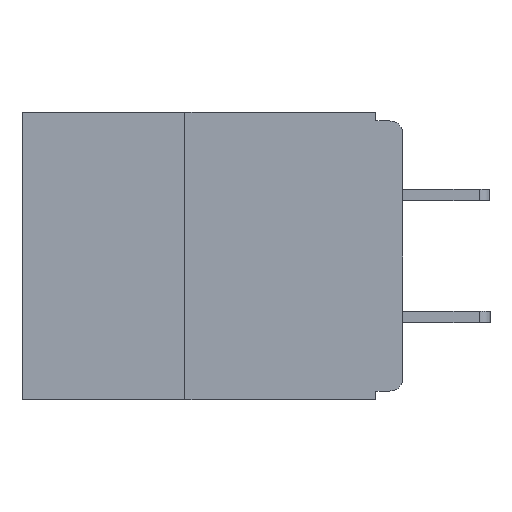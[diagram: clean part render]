
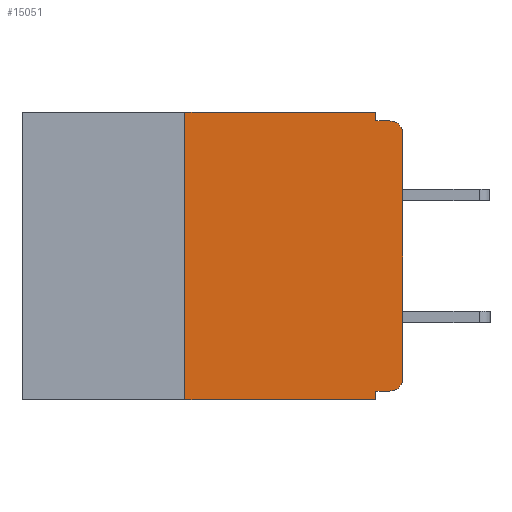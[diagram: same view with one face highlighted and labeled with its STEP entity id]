
A CAD part, left-side view. The second image highlights one B-rep face of the part: STEP entity #15051.
In plain terms, the highlighted planar face has unit normal (-1, 0, 0).
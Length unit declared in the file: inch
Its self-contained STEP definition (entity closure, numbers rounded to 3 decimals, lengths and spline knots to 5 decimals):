
#332 = CARTESIAN_POINT ( 'NONE',  ( 0., 0.031, -0.33 ) ) ;
#505 = CARTESIAN_POINT ( 'NONE',  ( 0., 0.015, -0.01 ) ) ;
#1168 = CARTESIAN_POINT ( 'NONE',  ( 0., 0.031, 0. ) ) ;
#1361 = ORIENTED_EDGE ( 'NONE', *, *, #12454, .T. ) ;
#1710 = VECTOR ( 'NONE', #12046, 39.37008 ) ;
#1731 = DIRECTION ( 'NONE',  ( -1., 0., 0. ) ) ;
#2186 = DIRECTION ( 'NONE',  ( 0., -1., 0. ) ) ;
#2817 = VERTEX_POINT ( 'NONE', #505 ) ;
#2874 = EDGE_CURVE ( 'NONE', #10611, #2817, #9341, .T. ) ;
#2976 = VERTEX_POINT ( 'NONE', #8326 ) ;
#3410 = LINE ( 'NONE', #15241, #10658 ) ;
#3461 = EDGE_CURVE ( 'NONE', #7447, #2817, #19648, .T. ) ;
#3481 = LINE ( 'NONE', #17397, #15344 ) ;
#3665 = CARTESIAN_POINT ( 'NONE',  ( 0., 0.25, 0. ) ) ;
#4322 = VERTEX_POINT ( 'NONE', #332 ) ;
#5037 = ORIENTED_EDGE ( 'NONE', *, *, #19252, .F. ) ;
#5082 = VECTOR ( 'NONE', #9387, 39.37008 ) ;
#5200 = LINE ( 'NONE', #10723, #17069 ) ;
#5267 = CARTESIAN_POINT ( 'NONE',  ( 0., 0.031, -0.33 ) ) ;
#5450 = CARTESIAN_POINT ( 'NONE',  ( 0., 0., -0.01 ) ) ;
#5561 = LINE ( 'NONE', #17117, #5082 ) ;
#5751 = EDGE_CURVE ( 'NONE', #2976, #15133, #3481, .T. ) ;
#5783 = VERTEX_POINT ( 'NONE', #3665 ) ;
#6056 = EDGE_CURVE ( 'NONE', #7244, #7447, #14625, .T. ) ;
#6333 = ORIENTED_EDGE ( 'NONE', *, *, #8469, .T. ) ;
#6437 = ORIENTED_EDGE ( 'NONE', *, *, #15261, .F. ) ;
#6460 = CARTESIAN_POINT ( 'NONE',  ( 0., 0., 0. ) ) ;
#6567 = CARTESIAN_POINT ( 'NONE',  ( 0., 0., -0.305 ) ) ;
#6750 = LINE ( 'NONE', #6460, #14561 ) ;
#6939 = ORIENTED_EDGE ( 'NONE', *, *, #3461, .F. ) ;
#7207 = CARTESIAN_POINT ( 'NONE',  ( 0., 0.031, 0. ) ) ;
#7244 = VERTEX_POINT ( 'NONE', #7207 ) ;
#7447 = VERTEX_POINT ( 'NONE', #18768 ) ;
#7630 = EDGE_CURVE ( 'NONE', #15133, #4322, #10176, .T. ) ;
#8180 = VERTEX_POINT ( 'NONE', #6567 ) ;
#8290 = AXIS2_PLACEMENT_3D ( 'NONE', #13359, #8723, #19452 ) ;
#8326 = CARTESIAN_POINT ( 'NONE',  ( 0., 0.015, -0.32 ) ) ;
#8469 = EDGE_CURVE ( 'NONE', #2976, #8180, #19533, .T. ) ;
#8721 = AXIS2_PLACEMENT_3D ( 'NONE', #19650, #13366, #12940 ) ;
#8723 = DIRECTION ( 'NONE',  ( 1., 0., 0. ) ) ;
#9241 = DIRECTION ( 'NONE',  ( 0., -1., 0. ) ) ;
#9341 = CIRCLE ( 'NONE', #8721, 0.015 ) ;
#9387 = DIRECTION ( 'NONE',  ( 0., -1., 0. ) ) ;
#10122 = ORIENTED_EDGE ( 'NONE', *, *, #6056, .F. ) ;
#10176 = LINE ( 'NONE', #5267, #17919 ) ;
#10611 = VERTEX_POINT ( 'NONE', #11671 ) ;
#10658 = VECTOR ( 'NONE', #13711, 39.37008 ) ;
#10723 = CARTESIAN_POINT ( 'NONE',  ( 0., 0.437, 0. ) ) ;
#11034 = CARTESIAN_POINT ( 'NONE',  ( 0., 0.015, -0.305 ) ) ;
#11171 = DIRECTION ( 'NONE',  ( 0., 0., 1. ) ) ;
#11434 = DIRECTION ( 'NONE',  ( 0., 0., -1. ) ) ;
#11671 = CARTESIAN_POINT ( 'NONE',  ( 0., 0., -0.025 ) ) ;
#12046 = DIRECTION ( 'NONE',  ( 0., 0., -1. ) ) ;
#12454 = EDGE_CURVE ( 'NONE', #15502, #4322, #5561, .T. ) ;
#12639 = DIRECTION ( 'NONE',  ( 0., 0., -1. ) ) ;
#12746 = DIRECTION ( 'NONE',  ( 0., 1., 0. ) ) ;
#12927 = CARTESIAN_POINT ( 'NONE',  ( 0., 0.25, -0.33 ) ) ;
#12940 = DIRECTION ( 'NONE',  ( 0., 0., -1. ) ) ;
#13359 = CARTESIAN_POINT ( 'NONE',  ( 0., 0.437, 0. ) ) ;
#13366 = DIRECTION ( 'NONE',  ( -1., 0., 0. ) ) ;
#13711 = DIRECTION ( 'NONE',  ( 0., 0., 1. ) ) ;
#14015 = ORIENTED_EDGE ( 'NONE', *, *, #7630, .F. ) ;
#14517 = EDGE_LOOP ( 'NONE', ( #19270, #16187, #6939, #10122, #6437, #5037, #1361, #14015, #19026, #6333 ) ) ;
#14561 = VECTOR ( 'NONE', #11171, 39.37008 ) ;
#14625 = LINE ( 'NONE', #1168, #1710 ) ;
#15051 = ADVANCED_FACE ( 'NONE', ( #16851 ), #16428, .F. ) ;
#15133 = VERTEX_POINT ( 'NONE', #16631 ) ;
#15153 = VECTOR ( 'NONE', #2186, 39.37008 ) ;
#15241 = CARTESIAN_POINT ( 'NONE',  ( 0., 0.25, -0.33 ) ) ;
#15261 = EDGE_CURVE ( 'NONE', #5783, #7244, #5200, .T. ) ;
#15344 = VECTOR ( 'NONE', #12746, 39.37008 ) ;
#15502 = VERTEX_POINT ( 'NONE', #12927 ) ;
#16187 = ORIENTED_EDGE ( 'NONE', *, *, #2874, .T. ) ;
#16428 = PLANE ( 'NONE',  #8290 ) ;
#16631 = CARTESIAN_POINT ( 'NONE',  ( 0., 0.031, -0.32 ) ) ;
#16851 = FACE_OUTER_BOUND ( 'NONE', #14517, .T. ) ;
#17069 = VECTOR ( 'NONE', #9241, 39.37008 ) ;
#17117 = CARTESIAN_POINT ( 'NONE',  ( 0., 0.437, -0.33 ) ) ;
#17397 = CARTESIAN_POINT ( 'NONE',  ( 0., 0., -0.32 ) ) ;
#17919 = VECTOR ( 'NONE', #11434, 39.37008 ) ;
#17974 = AXIS2_PLACEMENT_3D ( 'NONE', #11034, #1731, #12639 ) ;
#18768 = CARTESIAN_POINT ( 'NONE',  ( 0., 0.031, -0.01 ) ) ;
#18859 = EDGE_CURVE ( 'NONE', #8180, #10611, #6750, .T. ) ;
#19026 = ORIENTED_EDGE ( 'NONE', *, *, #5751, .F. ) ;
#19252 = EDGE_CURVE ( 'NONE', #15502, #5783, #3410, .T. ) ;
#19270 = ORIENTED_EDGE ( 'NONE', *, *, #18859, .T. ) ;
#19452 = DIRECTION ( 'NONE',  ( 0., 0., -1. ) ) ;
#19533 = CIRCLE ( 'NONE', #17974, 0.015 ) ;
#19648 = LINE ( 'NONE', #5450, #15153 ) ;
#19650 = CARTESIAN_POINT ( 'NONE',  ( 0., 0.015, -0.025 ) ) ;
